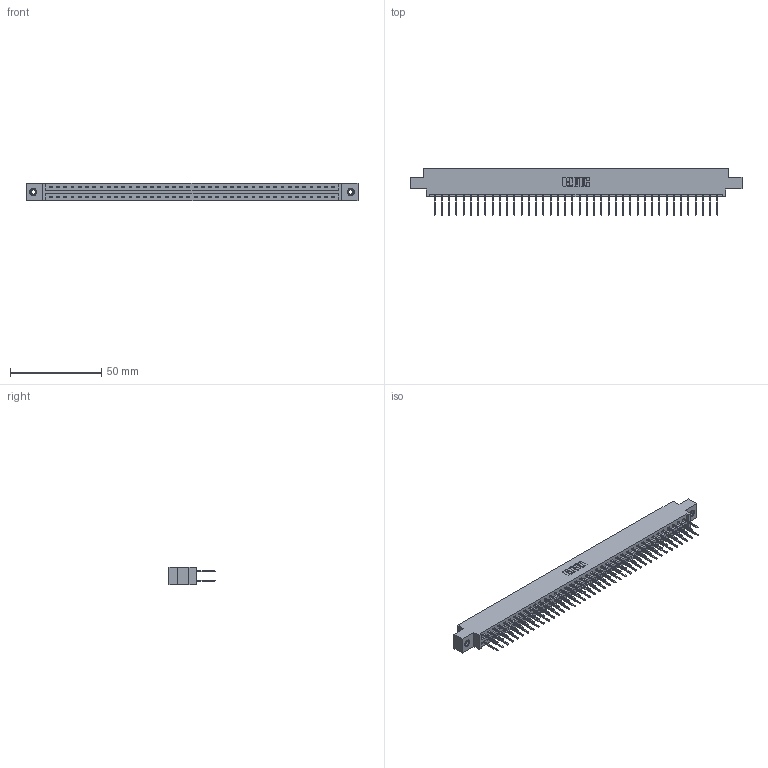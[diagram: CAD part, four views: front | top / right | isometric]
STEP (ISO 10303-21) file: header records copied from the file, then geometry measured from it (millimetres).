
FILE_DESCRIPTION (( 'STEP AP203' ), '1' );
FILE_NAME ('387-080-523-807.STEP', '2019-10-22T08:03:54', ( '' ), ( '' ), 'SwSTEP 2.0', 'SolidWorks 2016', '' );
FILE_SCHEMA (( 'CONFIG_CONTROL_DESIGN' ));
Length unit declared in the file: inch
Products named in the file (4): 345-292-001_345-293-123; 387-080-523-807; 345-250-001_345-250-005-103; 337 Part_0.170 Offset - 0.156 Dia-TI
Assembly tree (83 placements, depth 2):
  387-080-523-807
    337 Part_0.170 Offset - 0.156 Dia-TI
    345-292-001_345-293-123  x80
    345-250-001_345-250-005-103  x2
Bounding box: 181.51 x 25.15 x 9.4 mm (x, y, z)
Volume: 19135.1 mm3; surface area: 22535.9 mm2
Topology: 83 solids, 83 shells, 4498 faces, 13339 edges, 8778 vertices
Faces by surface type: plane 3146, cylinder 1336, cone 12, torus 4
Entity records: 32608 total; most frequent: CARTESIAN_POINT 5477, ORIENTED_EDGE 5406, DIRECTION 4693, EDGE_CURVE 2703, LINE 2555, VECTOR 2555, VERTEX_POINT 1796, AXIS2_PLACEMENT_3D 1069
